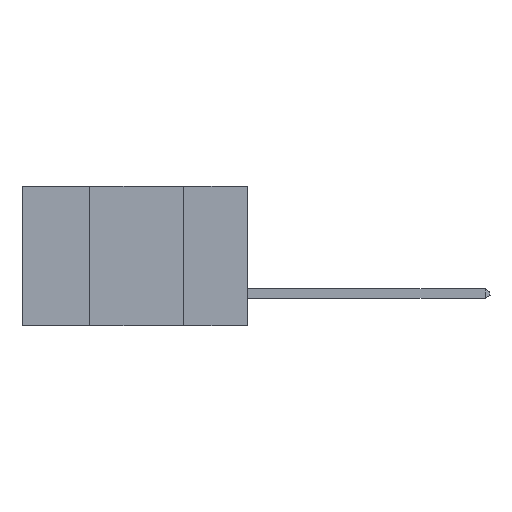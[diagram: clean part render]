
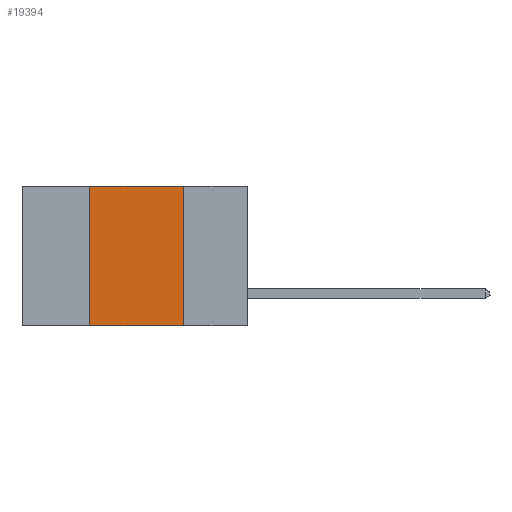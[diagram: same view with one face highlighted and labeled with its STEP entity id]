
A CAD part, left-side view. The second image highlights one B-rep face of the part: STEP entity #19394.
In plain terms, the highlighted planar face has unit normal (-1, 0, 0).
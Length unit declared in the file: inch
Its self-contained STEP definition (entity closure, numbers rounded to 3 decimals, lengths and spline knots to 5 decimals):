
#140 = ORIENTED_EDGE ( 'NONE', *, *, #15165, .F. ) ;
#186 = CARTESIAN_POINT ( 'NONE',  ( 0., 0.17, 0. ) ) ;
#1172 = LINE ( 'NONE', #8927, #23468 ) ;
#3331 = DIRECTION ( 'NONE',  ( 0., 0., -1. ) ) ;
#3433 = DIRECTION ( 'NONE',  ( 0., -1., 0. ) ) ;
#4917 = CARTESIAN_POINT ( 'NONE',  ( 0., 0.17, -0.37 ) ) ;
#7399 = ORIENTED_EDGE ( 'NONE', *, *, #14492, .T. ) ;
#7793 = EDGE_CURVE ( 'NONE', #15092, #15001, #23073, .T. ) ;
#8911 = DIRECTION ( 'NONE',  ( 1., 0., 0. ) ) ;
#8927 = CARTESIAN_POINT ( 'NONE',  ( 0., 0.6, -0.37 ) ) ;
#10025 = EDGE_CURVE ( 'NONE', #12244, #11496, #20690, .T. ) ;
#11496 = VERTEX_POINT ( 'NONE', #19067 ) ;
#12244 = VERTEX_POINT ( 'NONE', #15433 ) ;
#13080 = VECTOR ( 'NONE', #15505, 39.37008 ) ;
#13342 = LINE ( 'NONE', #13479, #13080 ) ;
#13479 = CARTESIAN_POINT ( 'NONE',  ( 0., 0.6, 0. ) ) ;
#14492 = EDGE_CURVE ( 'NONE', #12244, #15001, #1172, .T. ) ;
#14523 = PLANE ( 'NONE',  #20136 ) ;
#15001 = VERTEX_POINT ( 'NONE', #4917 ) ;
#15041 = DIRECTION ( 'NONE',  ( 0., 0., -1. ) ) ;
#15092 = VERTEX_POINT ( 'NONE', #23793 ) ;
#15165 = EDGE_CURVE ( 'NONE', #11496, #15092, #13342, .T. ) ;
#15433 = CARTESIAN_POINT ( 'NONE',  ( 0., 0.42, -0.37 ) ) ;
#15436 = ORIENTED_EDGE ( 'NONE', *, *, #7793, .F. ) ;
#15505 = DIRECTION ( 'NONE',  ( 0., -1., 0. ) ) ;
#18072 = VECTOR ( 'NONE', #18078, 39.37008 ) ;
#18078 = DIRECTION ( 'NONE',  ( 0., 0., 1. ) ) ;
#19067 = CARTESIAN_POINT ( 'NONE',  ( 0., 0.42, 0. ) ) ;
#19394 = ADVANCED_FACE ( 'NONE', ( #20714 ), #14523, .F. ) ;
#19610 = CARTESIAN_POINT ( 'NONE',  ( 0., 0.42, 0. ) ) ;
#20136 = AXIS2_PLACEMENT_3D ( 'NONE', #21629, #8911, #3331 ) ;
#20690 = LINE ( 'NONE', #19610, #18072 ) ;
#20714 = FACE_OUTER_BOUND ( 'NONE', #20905, .T. ) ;
#20905 = EDGE_LOOP ( 'NONE', ( #15436, #140, #21160, #7399 ) ) ;
#21160 = ORIENTED_EDGE ( 'NONE', *, *, #10025, .F. ) ;
#21333 = VECTOR ( 'NONE', #15041, 39.37008 ) ;
#21629 = CARTESIAN_POINT ( 'NONE',  ( 0., 0.6, 0. ) ) ;
#23073 = LINE ( 'NONE', #186, #21333 ) ;
#23468 = VECTOR ( 'NONE', #3433, 39.37008 ) ;
#23793 = CARTESIAN_POINT ( 'NONE',  ( 0., 0.17, 0. ) ) ;
